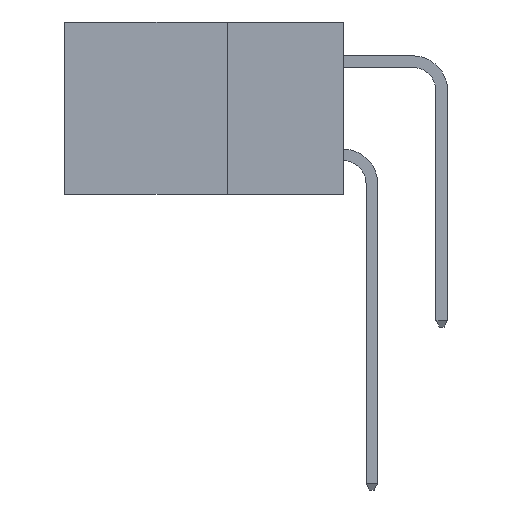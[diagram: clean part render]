
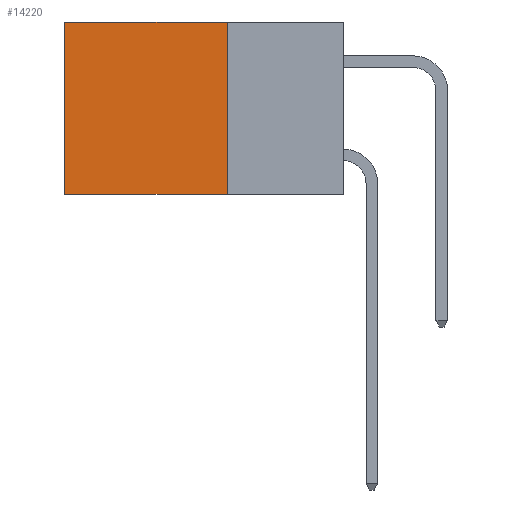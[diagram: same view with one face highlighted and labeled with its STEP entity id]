
A CAD part, left-side view. The second image highlights one B-rep face of the part: STEP entity #14220.
In plain terms, the highlighted planar face has unit normal (-1, 0, 0).
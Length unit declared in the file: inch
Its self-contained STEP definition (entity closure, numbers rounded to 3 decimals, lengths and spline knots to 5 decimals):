
#295 = VERTEX_POINT ( 'NONE', #13167 ) ;
#725 = DIRECTION ( 'NONE',  ( 1., 0., 0. ) ) ;
#746 = DIRECTION ( 'NONE',  ( 0., 0., -1. ) ) ;
#993 = VECTOR ( 'NONE', #17731, 39.37008 ) ;
#1521 = CARTESIAN_POINT ( 'NONE',  ( 0.2615, 0.25, 0. ) ) ;
#2523 = ORIENTED_EDGE ( 'NONE', *, *, #6439, .F. ) ;
#2769 = LINE ( 'NONE', #8714, #8969 ) ;
#2901 = CARTESIAN_POINT ( 'NONE',  ( 0.2615, 0.25, 0. ) ) ;
#3917 = EDGE_LOOP ( 'NONE', ( #15084, #2523, #9684, #9382 ) ) ;
#5909 = VECTOR ( 'NONE', #746, 39.37008 ) ;
#6439 = EDGE_CURVE ( 'NONE', #7372, #295, #2769, .T. ) ;
#6475 = VERTEX_POINT ( 'NONE', #1521 ) ;
#6930 = EDGE_CURVE ( 'NONE', #6475, #16582, #16023, .T. ) ;
#7372 = VERTEX_POINT ( 'NONE', #14709 ) ;
#7906 = CARTESIAN_POINT ( 'NONE',  ( 0.2615, 0.6, -0.37 ) ) ;
#8134 = LINE ( 'NONE', #7906, #15246 ) ;
#8714 = CARTESIAN_POINT ( 'NONE',  ( 0.2615, 0.25, -0.37 ) ) ;
#8969 = VECTOR ( 'NONE', #9231, 39.37008 ) ;
#9231 = DIRECTION ( 'NONE',  ( 0., 1., 0. ) ) ;
#9352 = DIRECTION ( 'NONE',  ( 0., 0., -1. ) ) ;
#9382 = ORIENTED_EDGE ( 'NONE', *, *, #6930, .T. ) ;
#9684 = ORIENTED_EDGE ( 'NONE', *, *, #13537, .F. ) ;
#10645 = DIRECTION ( 'NONE',  ( 0., 0., -1. ) ) ;
#11465 = FACE_OUTER_BOUND ( 'NONE', #3917, .T. ) ;
#11494 = EDGE_CURVE ( 'NONE', #16582, #295, #8134, .T. ) ;
#13167 = CARTESIAN_POINT ( 'NONE',  ( 0.2615, 0.6, -0.37 ) ) ;
#13537 = EDGE_CURVE ( 'NONE', #6475, #7372, #17173, .T. ) ;
#13896 = CARTESIAN_POINT ( 'NONE',  ( 0.2615, 0.6, 0. ) ) ;
#13963 = AXIS2_PLACEMENT_3D ( 'NONE', #17605, #725, #10645 ) ;
#14220 = ADVANCED_FACE ( 'NONE', ( #11465 ), #16226, .F. ) ;
#14709 = CARTESIAN_POINT ( 'NONE',  ( 0.2615, 0.25, -0.37 ) ) ;
#15084 = ORIENTED_EDGE ( 'NONE', *, *, #11494, .T. ) ;
#15246 = VECTOR ( 'NONE', #9352, 39.37008 ) ;
#16023 = LINE ( 'NONE', #2901, #993 ) ;
#16226 = PLANE ( 'NONE',  #13963 ) ;
#16582 = VERTEX_POINT ( 'NONE', #13896 ) ;
#17173 = LINE ( 'NONE', #17632, #5909 ) ;
#17605 = CARTESIAN_POINT ( 'NONE',  ( 0.2615, 0.25, -0.37 ) ) ;
#17632 = CARTESIAN_POINT ( 'NONE',  ( 0.2615, 0.25, -0.37 ) ) ;
#17731 = DIRECTION ( 'NONE',  ( 0., 1., 0. ) ) ;
